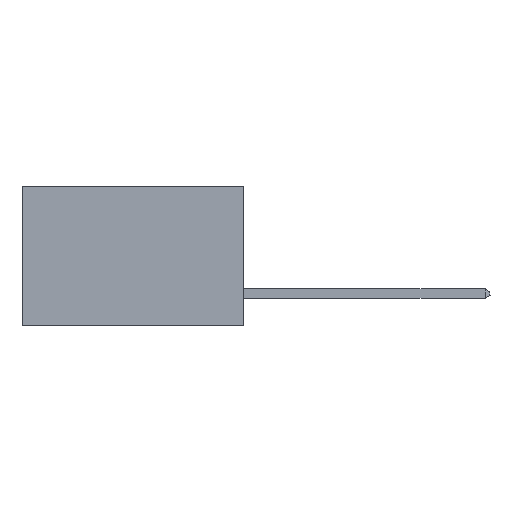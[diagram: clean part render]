
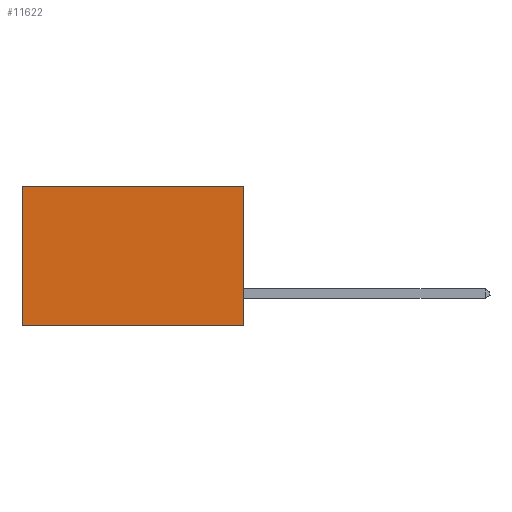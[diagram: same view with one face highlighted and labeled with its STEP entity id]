
A CAD part, left-side view. The second image highlights one B-rep face of the part: STEP entity #11622.
In plain terms, the highlighted planar face has unit normal (-1, 0, 0).
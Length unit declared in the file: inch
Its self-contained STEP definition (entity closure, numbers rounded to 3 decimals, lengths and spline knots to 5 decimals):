
#895 = DIRECTION ( 'NONE',  ( 0., 0., -1. ) ) ;
#1156 = CARTESIAN_POINT ( 'NONE',  ( 0.277, 0., 0. ) ) ;
#1247 = DIRECTION ( 'NONE',  ( 0., 1., 0. ) ) ;
#1295 = EDGE_LOOP ( 'NONE', ( #29081, #9463, #15327, #12242 ) ) ;
#2201 = VECTOR ( 'NONE', #1247, 39.37008 ) ;
#2503 = LINE ( 'NONE', #13319, #7335 ) ;
#3022 = CARTESIAN_POINT ( 'NONE',  ( 0.277, 0.59, 0. ) ) ;
#3992 = EDGE_CURVE ( 'NONE', #29695, #20621, #21328, .T. ) ;
#7335 = VECTOR ( 'NONE', #18208, 39.37008 ) ;
#7382 = CARTESIAN_POINT ( 'NONE',  ( 0.277, 0.59, -0.37 ) ) ;
#7912 = DIRECTION ( 'NONE',  ( 0., 0., -1. ) ) ;
#9463 = ORIENTED_EDGE ( 'NONE', *, *, #14849, .F. ) ;
#9615 = DIRECTION ( 'NONE',  ( 0., 0., -1. ) ) ;
#10599 = EDGE_CURVE ( 'NONE', #20621, #20527, #25294, .T. ) ;
#10858 = VECTOR ( 'NONE', #7912, 39.37008 ) ;
#11622 = ADVANCED_FACE ( 'NONE', ( #30462 ), #21681, .F. ) ;
#11898 = CARTESIAN_POINT ( 'NONE',  ( 0.277, 0., -0.37 ) ) ;
#12242 = ORIENTED_EDGE ( 'NONE', *, *, #3992, .T. ) ;
#13319 = CARTESIAN_POINT ( 'NONE',  ( 0.277, 0., -0.37 ) ) ;
#14849 = EDGE_CURVE ( 'NONE', #23043, #20527, #2503, .T. ) ;
#15327 = ORIENTED_EDGE ( 'NONE', *, *, #29086, .F. ) ;
#17617 = CARTESIAN_POINT ( 'NONE',  ( 0.277, 0., -0.37 ) ) ;
#17680 = VECTOR ( 'NONE', #895, 39.37008 ) ;
#18208 = DIRECTION ( 'NONE',  ( 0., 1., 0. ) ) ;
#19678 = CARTESIAN_POINT ( 'NONE',  ( 0.277, 0., 0. ) ) ;
#19882 = CARTESIAN_POINT ( 'NONE',  ( 0.277, 0.59, -0.37 ) ) ;
#20527 = VERTEX_POINT ( 'NONE', #7382 ) ;
#20621 = VERTEX_POINT ( 'NONE', #3022 ) ;
#20750 = AXIS2_PLACEMENT_3D ( 'NONE', #11898, #24127, #9615 ) ;
#21328 = LINE ( 'NONE', #1156, #2201 ) ;
#21681 = PLANE ( 'NONE',  #20750 ) ;
#23043 = VERTEX_POINT ( 'NONE', #26018 ) ;
#24127 = DIRECTION ( 'NONE',  ( 1., 0., 0. ) ) ;
#25294 = LINE ( 'NONE', #19882, #10858 ) ;
#26018 = CARTESIAN_POINT ( 'NONE',  ( 0.277, 0., -0.37 ) ) ;
#29081 = ORIENTED_EDGE ( 'NONE', *, *, #10599, .T. ) ;
#29086 = EDGE_CURVE ( 'NONE', #29695, #23043, #29771, .T. ) ;
#29695 = VERTEX_POINT ( 'NONE', #19678 ) ;
#29771 = LINE ( 'NONE', #17617, #17680 ) ;
#30462 = FACE_OUTER_BOUND ( 'NONE', #1295, .T. ) ;
